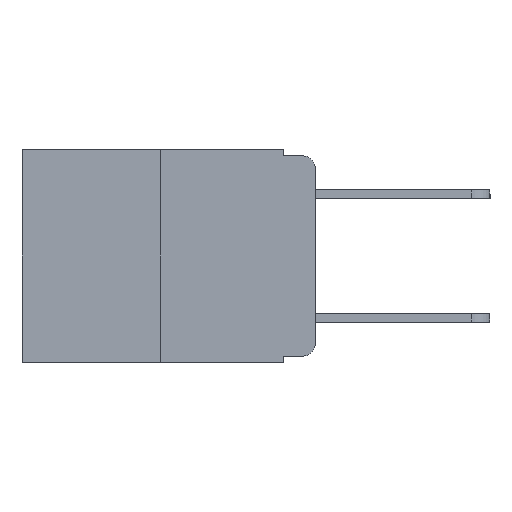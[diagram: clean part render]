
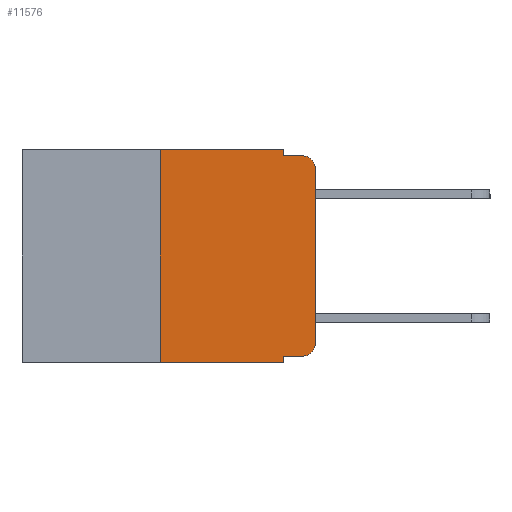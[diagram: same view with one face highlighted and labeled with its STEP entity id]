
A CAD part, left-side view. The second image highlights one B-rep face of the part: STEP entity #11576.
In plain terms, the highlighted planar face has unit normal (-1, 0, 0).
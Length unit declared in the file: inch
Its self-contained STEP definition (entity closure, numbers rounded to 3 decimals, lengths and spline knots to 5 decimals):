
#227 = VECTOR ( 'NONE', #2472, 39.37008 ) ;
#346 = ORIENTED_EDGE ( 'NONE', *, *, #5838, .T. ) ;
#375 = ORIENTED_EDGE ( 'NONE', *, *, #5365, .F. ) ;
#544 = ORIENTED_EDGE ( 'NONE', *, *, #4696, .T. ) ;
#630 = CARTESIAN_POINT ( 'NONE',  ( 0., 0.051, -0.333 ) ) ;
#779 = CARTESIAN_POINT ( 'NONE',  ( 0., 0.051, -0.333 ) ) ;
#929 = ORIENTED_EDGE ( 'NONE', *, *, #9894, .F. ) ;
#995 = ORIENTED_EDGE ( 'NONE', *, *, #10961, .F. ) ;
#1226 = DIRECTION ( 'NONE',  ( 0., 0., -1. ) ) ;
#1439 = CARTESIAN_POINT ( 'NONE',  ( 0., 0.051, 0. ) ) ;
#1506 = VERTEX_POINT ( 'NONE', #10904 ) ;
#1734 = AXIS2_PLACEMENT_3D ( 'NONE', #10409, #11155, #6326 ) ;
#1831 = ORIENTED_EDGE ( 'NONE', *, *, #9344, .F. ) ;
#2127 = AXIS2_PLACEMENT_3D ( 'NONE', #7699, #7688, #7678 ) ;
#2222 = AXIS2_PLACEMENT_3D ( 'NONE', #8220, #5931, #7284 ) ;
#2297 = CIRCLE ( 'NONE', #2127, 0.02 ) ;
#2314 = LINE ( 'NONE', #9690, #4903 ) ;
#2472 = DIRECTION ( 'NONE',  ( 0., -1., 0. ) ) ;
#2679 = LINE ( 'NONE', #8780, #5219 ) ;
#2744 = VERTEX_POINT ( 'NONE', #7272 ) ;
#3001 = VERTEX_POINT ( 'NONE', #4480 ) ;
#3028 = ORIENTED_EDGE ( 'NONE', *, *, #8391, .F. ) ;
#3157 = VECTOR ( 'NONE', #1226, 39.37008 ) ;
#3628 = LINE ( 'NONE', #5562, #10392 ) ;
#3662 = VECTOR ( 'NONE', #11834, 39.37008 ) ;
#3688 = VERTEX_POINT ( 'NONE', #6217 ) ;
#3696 = EDGE_LOOP ( 'NONE', ( #4505, #4541, #3028, #1831, #375, #995, #346, #929, #544, #5207 ) ) ;
#3768 = CIRCLE ( 'NONE', #2222, 0.02 ) ;
#3944 = VERTEX_POINT ( 'NONE', #11283 ) ;
#4091 = CARTESIAN_POINT ( 'NONE',  ( 0., 0.02, -0.333 ) ) ;
#4231 = VECTOR ( 'NONE', #9946, 39.37008 ) ;
#4480 = CARTESIAN_POINT ( 'NONE',  ( 0., 0.02, -0.01 ) ) ;
#4505 = ORIENTED_EDGE ( 'NONE', *, *, #8090, .T. ) ;
#4541 = ORIENTED_EDGE ( 'NONE', *, *, #8409, .T. ) ;
#4696 = EDGE_CURVE ( 'NONE', #7811, #6507, #8337, .T. ) ;
#4746 = VERTEX_POINT ( 'NONE', #6336 ) ;
#4903 = VECTOR ( 'NONE', #9678, 39.37008 ) ;
#5207 = ORIENTED_EDGE ( 'NONE', *, *, #7550, .T. ) ;
#5219 = VECTOR ( 'NONE', #8751, 39.37008 ) ;
#5229 = DIRECTION ( 'NONE',  ( 0., -1., 0. ) ) ;
#5365 = EDGE_CURVE ( 'NONE', #4746, #7624, #11570, .T. ) ;
#5562 = CARTESIAN_POINT ( 'NONE',  ( 0., 0.473, -0.343 ) ) ;
#5838 = EDGE_CURVE ( 'NONE', #2744, #3688, #3628, .T. ) ;
#5913 = LINE ( 'NONE', #1439, #3157 ) ;
#5931 = DIRECTION ( 'NONE',  ( -1., 0., 0. ) ) ;
#6217 = CARTESIAN_POINT ( 'NONE',  ( 0., 0.051, -0.343 ) ) ;
#6326 = DIRECTION ( 'NONE',  ( 0., 0., -1. ) ) ;
#6336 = CARTESIAN_POINT ( 'NONE',  ( 0., 0.25, 0. ) ) ;
#6507 = VERTEX_POINT ( 'NONE', #4091 ) ;
#7080 = VECTOR ( 'NONE', #9771, 39.37008 ) ;
#7272 = CARTESIAN_POINT ( 'NONE',  ( 0., 0.25, -0.343 ) ) ;
#7284 = DIRECTION ( 'NONE',  ( 0., 0., -1. ) ) ;
#7550 = EDGE_CURVE ( 'NONE', #6507, #3944, #3768, .T. ) ;
#7624 = VERTEX_POINT ( 'NONE', #10188 ) ;
#7678 = DIRECTION ( 'NONE',  ( 0., 0., -1. ) ) ;
#7688 = DIRECTION ( 'NONE',  ( -1., 0., 0. ) ) ;
#7699 = CARTESIAN_POINT ( 'NONE',  ( 0., 0.02, -0.03 ) ) ;
#7811 = VERTEX_POINT ( 'NONE', #779 ) ;
#7949 = CARTESIAN_POINT ( 'NONE',  ( 0., 0.25, 0. ) ) ;
#8010 = CARTESIAN_POINT ( 'NONE',  ( 0., 0., -0.03 ) ) ;
#8090 = EDGE_CURVE ( 'NONE', #3944, #9453, #2314, .T. ) ;
#8220 = CARTESIAN_POINT ( 'NONE',  ( 0., 0.02, -0.313 ) ) ;
#8337 = LINE ( 'NONE', #630, #227 ) ;
#8391 = EDGE_CURVE ( 'NONE', #1506, #3001, #2679, .T. ) ;
#8409 = EDGE_CURVE ( 'NONE', #9453, #3001, #2297, .T. ) ;
#8751 = DIRECTION ( 'NONE',  ( 0., -1., 0. ) ) ;
#8780 = CARTESIAN_POINT ( 'NONE',  ( 0., 0.051, -0.01 ) ) ;
#8811 = LINE ( 'NONE', #7949, #3662 ) ;
#8975 = LINE ( 'NONE', #9007, #4231 ) ;
#9007 = CARTESIAN_POINT ( 'NONE',  ( 0., 0.051, 0. ) ) ;
#9344 = EDGE_CURVE ( 'NONE', #7624, #1506, #8975, .T. ) ;
#9453 = VERTEX_POINT ( 'NONE', #8010 ) ;
#9620 = PLANE ( 'NONE',  #1734 ) ;
#9678 = DIRECTION ( 'NONE',  ( 0., 0., 1. ) ) ;
#9690 = CARTESIAN_POINT ( 'NONE',  ( 0., 0., 0. ) ) ;
#9771 = DIRECTION ( 'NONE',  ( 0., -1., 0. ) ) ;
#9800 = FACE_OUTER_BOUND ( 'NONE', #3696, .T. ) ;
#9831 = CARTESIAN_POINT ( 'NONE',  ( 0., 0.473, 0. ) ) ;
#9894 = EDGE_CURVE ( 'NONE', #7811, #3688, #5913, .T. ) ;
#9946 = DIRECTION ( 'NONE',  ( 0., 0., -1. ) ) ;
#10188 = CARTESIAN_POINT ( 'NONE',  ( 0., 0.051, 0. ) ) ;
#10392 = VECTOR ( 'NONE', #5229, 39.37008 ) ;
#10409 = CARTESIAN_POINT ( 'NONE',  ( 0., 0.473, 0. ) ) ;
#10904 = CARTESIAN_POINT ( 'NONE',  ( 0., 0.051, -0.01 ) ) ;
#10961 = EDGE_CURVE ( 'NONE', #2744, #4746, #8811, .T. ) ;
#11155 = DIRECTION ( 'NONE',  ( 1., 0., 0. ) ) ;
#11283 = CARTESIAN_POINT ( 'NONE',  ( 0., 0., -0.313 ) ) ;
#11570 = LINE ( 'NONE', #9831, #7080 ) ;
#11576 = ADVANCED_FACE ( 'NONE', ( #9800 ), #9620, .F. ) ;
#11834 = DIRECTION ( 'NONE',  ( 0., 0., 1. ) ) ;
